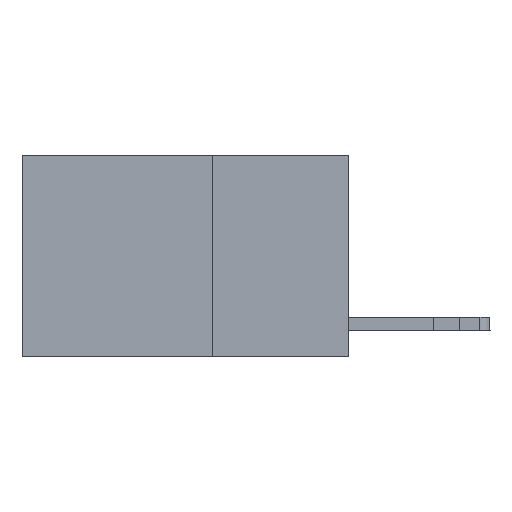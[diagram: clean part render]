
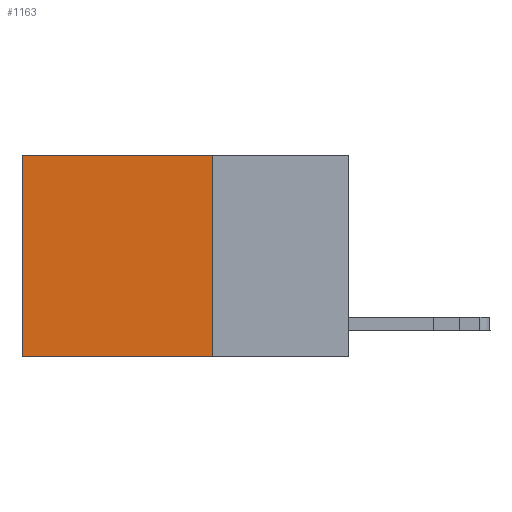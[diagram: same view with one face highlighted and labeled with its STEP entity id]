
A CAD part, left-side view. The second image highlights one B-rep face of the part: STEP entity #1163.
In plain terms, the highlighted planar face has unit normal (-1, 0, 0).
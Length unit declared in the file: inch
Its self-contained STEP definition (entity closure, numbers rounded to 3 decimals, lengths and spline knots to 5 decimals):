
#240 = CARTESIAN_POINT ( 'NONE',  ( 0.2625, 0.6, 0. ) ) ;
#384 = ORIENTED_EDGE ( 'NONE', *, *, #10866, .T. ) ;
#445 = LINE ( 'NONE', #11307, #12778 ) ;
#520 = VERTEX_POINT ( 'NONE', #882 ) ;
#569 = DIRECTION ( 'NONE',  ( 0., 1., 0. ) ) ;
#611 = FACE_OUTER_BOUND ( 'NONE', #12213, .T. ) ;
#757 = VECTOR ( 'NONE', #14913, 39.37008 ) ;
#827 = VECTOR ( 'NONE', #5795, 39.37008 ) ;
#882 = CARTESIAN_POINT ( 'NONE',  ( 0.2625, 0.25, 0. ) ) ;
#1163 = ADVANCED_FACE ( 'NONE', ( #611 ), #11535, .F. ) ;
#1169 = LINE ( 'NONE', #13828, #757 ) ;
#1444 = CARTESIAN_POINT ( 'NONE',  ( 0.2625, 0.25, -0.37 ) ) ;
#1473 = ORIENTED_EDGE ( 'NONE', *, *, #6467, .F. ) ;
#3470 = VERTEX_POINT ( 'NONE', #240 ) ;
#5795 = DIRECTION ( 'NONE',  ( 0., 0., -1. ) ) ;
#6467 = EDGE_CURVE ( 'NONE', #6813, #9749, #1169, .T. ) ;
#6677 = EDGE_CURVE ( 'NONE', #520, #6813, #10865, .T. ) ;
#6813 = VERTEX_POINT ( 'NONE', #1444 ) ;
#8326 = DIRECTION ( 'NONE',  ( 0., 0., -1. ) ) ;
#9749 = VERTEX_POINT ( 'NONE', #13291 ) ;
#9782 = ORIENTED_EDGE ( 'NONE', *, *, #9972, .T. ) ;
#9972 = EDGE_CURVE ( 'NONE', #520, #3470, #445, .T. ) ;
#10368 = LINE ( 'NONE', #11691, #827 ) ;
#10865 = LINE ( 'NONE', #13035, #13568 ) ;
#10866 = EDGE_CURVE ( 'NONE', #3470, #9749, #10368, .T. ) ;
#11307 = CARTESIAN_POINT ( 'NONE',  ( 0.2625, 0.25, 0. ) ) ;
#11363 = DIRECTION ( 'NONE',  ( 0., 0., -1. ) ) ;
#11409 = DIRECTION ( 'NONE',  ( 1., 0., 0. ) ) ;
#11520 = CARTESIAN_POINT ( 'NONE',  ( 0.2625, 0.25, 0. ) ) ;
#11535 = PLANE ( 'NONE',  #11660 ) ;
#11660 = AXIS2_PLACEMENT_3D ( 'NONE', #11520, #11409, #11363 ) ;
#11691 = CARTESIAN_POINT ( 'NONE',  ( 0.2625, 0.6, 0. ) ) ;
#12213 = EDGE_LOOP ( 'NONE', ( #384, #1473, #12701, #9782 ) ) ;
#12701 = ORIENTED_EDGE ( 'NONE', *, *, #6677, .F. ) ;
#12778 = VECTOR ( 'NONE', #569, 39.37008 ) ;
#13035 = CARTESIAN_POINT ( 'NONE',  ( 0.2625, 0.25, 0. ) ) ;
#13291 = CARTESIAN_POINT ( 'NONE',  ( 0.2625, 0.6, -0.37 ) ) ;
#13568 = VECTOR ( 'NONE', #8326, 39.37008 ) ;
#13828 = CARTESIAN_POINT ( 'NONE',  ( 0.2625, 0.25, -0.37 ) ) ;
#14913 = DIRECTION ( 'NONE',  ( 0., 1., 0. ) ) ;
